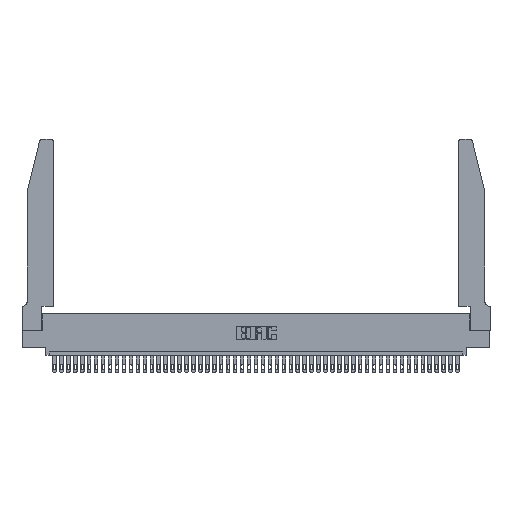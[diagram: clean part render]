
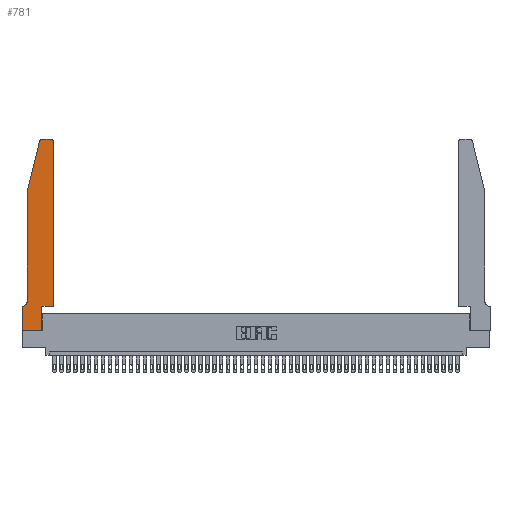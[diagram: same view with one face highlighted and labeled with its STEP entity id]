
A CAD part, top view. The second image highlights one B-rep face of the part: STEP entity #781.
In plain terms, the highlighted planar face has unit normal (0, 0, 1).
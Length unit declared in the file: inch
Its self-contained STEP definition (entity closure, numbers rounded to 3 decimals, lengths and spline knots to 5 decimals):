
#209 = DIRECTION ( 'NONE',  ( -1., 0., 0. ) ) ;
#443 = ORIENTED_EDGE ( 'NONE', *, *, #5368, .T. ) ;
#781 = ADVANCED_FACE ( 'NONE', ( #7572 ), #28354, .T. ) ;
#844 = CARTESIAN_POINT ( 'NONE',  ( 0.284, 2.75, 0.37 ) ) ;
#1462 = DIRECTION ( 'NONE',  ( 1., 0., 0. ) ) ;
#3367 = CARTESIAN_POINT ( 'NONE',  ( 0.0755, 2., 0.37 ) ) ;
#3575 = CARTESIAN_POINT ( 'NONE',  ( 0.4505, 0.35, 0.37 ) ) ;
#3899 = CARTESIAN_POINT ( 'NONE',  ( 0.0755, 2., 0.37 ) ) ;
#3943 = EDGE_CURVE ( 'NONE', #33657, #46198, #37860, .T. ) ;
#4205 = ORIENTED_EDGE ( 'NONE', *, *, #39601, .T. ) ;
#4855 = ORIENTED_EDGE ( 'NONE', *, *, #39447, .T. ) ;
#5317 = CARTESIAN_POINT ( 'NONE',  ( 0.4205, 2.72, 0.37 ) ) ;
#5351 = LINE ( 'NONE', #44290, #41554 ) ;
#5368 = EDGE_CURVE ( 'NONE', #6635, #18932, #22438, .T. ) ;
#5394 = VECTOR ( 'NONE', #21488, 39.37008 ) ;
#6635 = VERTEX_POINT ( 'NONE', #14082 ) ;
#7197 = VECTOR ( 'NONE', #21053, 39.37008 ) ;
#7572 = FACE_OUTER_BOUND ( 'NONE', #42667, .T. ) ;
#7820 = CARTESIAN_POINT ( 'NONE',  ( 0., 0.35, 0.37 ) ) ;
#8469 = EDGE_CURVE ( 'NONE', #17490, #16291, #9658, .T. ) ;
#8754 = CARTESIAN_POINT ( 'NONE',  ( 0.0055, 0.35, 0.37 ) ) ;
#9386 = LINE ( 'NONE', #11930, #44496 ) ;
#9658 = LINE ( 'NONE', #3899, #31155 ) ;
#11791 = CARTESIAN_POINT ( 'NONE',  ( 0.4505, 0.35, 0.37 ) ) ;
#11930 = CARTESIAN_POINT ( 'NONE',  ( 0., 0., 0.37 ) ) ;
#12460 = VECTOR ( 'NONE', #29045, 39.37008 ) ;
#13303 = CARTESIAN_POINT ( 'NONE',  ( 0., 0., 0.37 ) ) ;
#13365 = CARTESIAN_POINT ( 'NONE',  ( 0.2865, 0.35, 0.37 ) ) ;
#13566 = ORIENTED_EDGE ( 'NONE', *, *, #42177, .T. ) ;
#14059 = LINE ( 'NONE', #11791, #33319 ) ;
#14082 = CARTESIAN_POINT ( 'NONE',  ( 0.4505, 2.72, 0.37 ) ) ;
#14361 = VERTEX_POINT ( 'NONE', #844 ) ;
#15172 = LINE ( 'NONE', #41338, #23641 ) ;
#16291 = VERTEX_POINT ( 'NONE', #3367 ) ;
#16444 = ORIENTED_EDGE ( 'NONE', *, *, #45079, .T. ) ;
#16635 = EDGE_CURVE ( 'NONE', #26158, #33657, #29267, .T. ) ;
#17490 = VERTEX_POINT ( 'NONE', #36898 ) ;
#17557 = CARTESIAN_POINT ( 'NONE',  ( 0.4505, 0.35, 0.37 ) ) ;
#18932 = VERTEX_POINT ( 'NONE', #46179 ) ;
#19674 = DIRECTION ( 'NONE',  ( -1., 0., 0. ) ) ;
#21053 = DIRECTION ( 'NONE',  ( 1., 0., 0. ) ) ;
#21367 = DIRECTION ( 'NONE',  ( 0., 0., 1. ) ) ;
#21488 = DIRECTION ( 'NONE',  ( 0., 1., 0. ) ) ;
#22438 = CIRCLE ( 'NONE', #27041, 0.03 ) ;
#23134 = CARTESIAN_POINT ( 'NONE',  ( 0.284, 2.72, 0.37 ) ) ;
#23641 = VECTOR ( 'NONE', #19674, 39.37008 ) ;
#25949 = CARTESIAN_POINT ( 'NONE',  ( 0.2865, 0., 0.37 ) ) ;
#26066 = LINE ( 'NONE', #28410, #12460 ) ;
#26158 = VERTEX_POINT ( 'NONE', #40442 ) ;
#26586 = ORIENTED_EDGE ( 'NONE', *, *, #8469, .T. ) ;
#27041 = AXIS2_PLACEMENT_3D ( 'NONE', #5317, #30646, #27170 ) ;
#27170 = DIRECTION ( 'NONE',  ( 1., 0., 0. ) ) ;
#27947 = VERTEX_POINT ( 'NONE', #7820 ) ;
#28071 = CIRCLE ( 'NONE', #38505, 0.03 ) ;
#28354 = PLANE ( 'NONE',  #46067 ) ;
#28410 = CARTESIAN_POINT ( 'NONE',  ( 0.2605, 2.75, 0.37 ) ) ;
#29045 = DIRECTION ( 'NONE',  ( -1., 0., 0. ) ) ;
#29267 = LINE ( 'NONE', #13303, #7197 ) ;
#29768 = DIRECTION ( 'NONE',  ( 0., 1., 0. ) ) ;
#29868 = DIRECTION ( 'NONE',  ( 0., -1., 0. ) ) ;
#29927 = CARTESIAN_POINT ( 'NONE',  ( 0.2865, 0.35, 0.37 ) ) ;
#29956 = ORIENTED_EDGE ( 'NONE', *, *, #44983, .T. ) ;
#29970 = VECTOR ( 'NONE', #29768, 39.37008 ) ;
#30082 = AXIS2_PLACEMENT_3D ( 'NONE', #43736, #46773, #209 ) ;
#30206 = EDGE_CURVE ( 'NONE', #35859, #30587, #39711, .T. ) ;
#30587 = VERTEX_POINT ( 'NONE', #8754 ) ;
#30646 = DIRECTION ( 'NONE',  ( 0., 0., 1. ) ) ;
#31155 = VECTOR ( 'NONE', #32853, 39.37008 ) ;
#32297 = CARTESIAN_POINT ( 'NONE',  ( 0., 0.35, 0.37 ) ) ;
#32333 = CARTESIAN_POINT ( 'NONE',  ( 0.0755, 0.42, 0.37 ) ) ;
#32853 = DIRECTION ( 'NONE',  ( -0.239, -0.971, 0. ) ) ;
#33319 = VECTOR ( 'NONE', #40246, 39.37008 ) ;
#33657 = VERTEX_POINT ( 'NONE', #25949 ) ;
#33734 = DIRECTION ( 'NONE',  ( 0., -1., 0. ) ) ;
#34473 = ORIENTED_EDGE ( 'NONE', *, *, #42583, .T. ) ;
#35790 = ORIENTED_EDGE ( 'NONE', *, *, #41822, .T. ) ;
#35859 = VERTEX_POINT ( 'NONE', #32333 ) ;
#36898 = CARTESIAN_POINT ( 'NONE',  ( 0.25487, 2.72718, 0.37 ) ) ;
#37372 = ORIENTED_EDGE ( 'NONE', *, *, #16635, .T. ) ;
#37860 = LINE ( 'NONE', #29927, #29970 ) ;
#38505 = AXIS2_PLACEMENT_3D ( 'NONE', #23134, #44844, #1462 ) ;
#39219 = DIRECTION ( 'NONE',  ( 1., 0., 0. ) ) ;
#39447 = EDGE_CURVE ( 'NONE', #46198, #40443, #14059, .T. ) ;
#39601 = EDGE_CURVE ( 'NONE', #30587, #27947, #15172, .T. ) ;
#39711 = CIRCLE ( 'NONE', #30082, 0.07 ) ;
#40246 = DIRECTION ( 'NONE',  ( 1., 0., 0. ) ) ;
#40442 = CARTESIAN_POINT ( 'NONE',  ( 0., 0., 0.37 ) ) ;
#40443 = VERTEX_POINT ( 'NONE', #3575 ) ;
#41338 = CARTESIAN_POINT ( 'NONE',  ( 0.0755, 0.35, 0.37 ) ) ;
#41554 = VECTOR ( 'NONE', #29868, 39.37008 ) ;
#41822 = EDGE_CURVE ( 'NONE', #40443, #6635, #43932, .T. ) ;
#42177 = EDGE_CURVE ( 'NONE', #16291, #35859, #5351, .T. ) ;
#42583 = EDGE_CURVE ( 'NONE', #18932, #14361, #26066, .T. ) ;
#42667 = EDGE_LOOP ( 'NONE', ( #34473, #29956, #26586, #13566, #44581, #4205, #16444, #37372, #45016, #4855, #35790, #443 ) ) ;
#43736 = CARTESIAN_POINT ( 'NONE',  ( 0.0055, 0.42, 0.37 ) ) ;
#43932 = LINE ( 'NONE', #17557, #5394 ) ;
#44290 = CARTESIAN_POINT ( 'NONE',  ( 0.0755, 2., 0.37 ) ) ;
#44496 = VECTOR ( 'NONE', #33734, 39.37008 ) ;
#44581 = ORIENTED_EDGE ( 'NONE', *, *, #30206, .T. ) ;
#44844 = DIRECTION ( 'NONE',  ( 0., 0., 1. ) ) ;
#44983 = EDGE_CURVE ( 'NONE', #14361, #17490, #28071, .T. ) ;
#45016 = ORIENTED_EDGE ( 'NONE', *, *, #3943, .T. ) ;
#45079 = EDGE_CURVE ( 'NONE', #27947, #26158, #9386, .T. ) ;
#46067 = AXIS2_PLACEMENT_3D ( 'NONE', #32297, #21367, #39219 ) ;
#46179 = CARTESIAN_POINT ( 'NONE',  ( 0.4205, 2.75, 0.37 ) ) ;
#46198 = VERTEX_POINT ( 'NONE', #13365 ) ;
#46773 = DIRECTION ( 'NONE',  ( 0., 0., -1. ) ) ;
